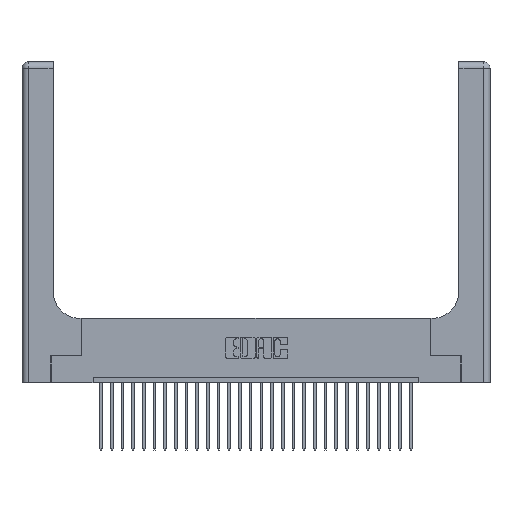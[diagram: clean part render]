
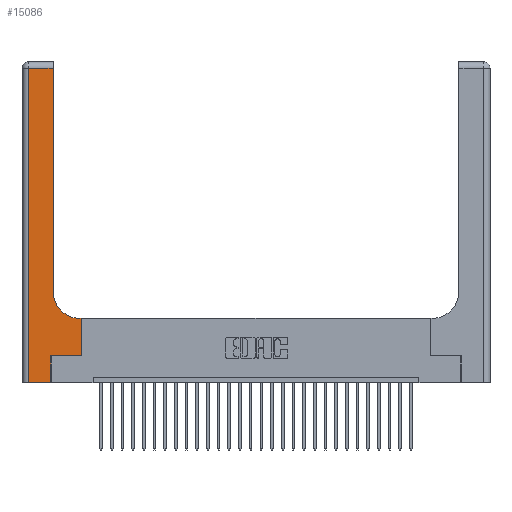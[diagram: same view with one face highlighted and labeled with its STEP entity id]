
A CAD part, top view. The second image highlights one B-rep face of the part: STEP entity #15086.
In plain terms, the highlighted planar face has unit normal (0, 0, 1).
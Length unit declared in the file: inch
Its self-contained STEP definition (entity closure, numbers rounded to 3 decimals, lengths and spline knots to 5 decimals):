
#100 = CARTESIAN_POINT ( 'NONE',  ( 0., 2.94, 0.37 ) ) ;
#261 = EDGE_CURVE ( 'NONE', #6286, #23740, #1936, .T. ) ;
#393 = DIRECTION ( 'NONE',  ( -1., 0., 0. ) ) ;
#439 = CARTESIAN_POINT ( 'NONE',  ( 0.5585, 0.6, 0.37 ) ) ;
#1012 = ORIENTED_EDGE ( 'NONE', *, *, #18084, .T. ) ;
#1936 = LINE ( 'NONE', #100, #5822 ) ;
#2536 = DIRECTION ( 'NONE',  ( 1., 0., 0. ) ) ;
#2660 = ORIENTED_EDGE ( 'NONE', *, *, #26138, .T. ) ;
#2692 = EDGE_CURVE ( 'NONE', #22903, #27558, #24898, .T. ) ;
#3680 = DIRECTION ( 'NONE',  ( -1., 0., 0. ) ) ;
#4266 = CARTESIAN_POINT ( 'NONE',  ( 0.269, 0., 0.37 ) ) ;
#4483 = EDGE_CURVE ( 'NONE', #23740, #28338, #14340, .T. ) ;
#4699 = DIRECTION ( 'NONE',  ( 0., 1., 0. ) ) ;
#4747 = EDGE_CURVE ( 'NONE', #27558, #6286, #4764, .T. ) ;
#4764 = LINE ( 'NONE', #18593, #23961 ) ;
#4982 = DIRECTION ( 'NONE',  ( -1., 0., 0. ) ) ;
#5817 = CARTESIAN_POINT ( 'NONE',  ( 0.2915, 0.85, 0.37 ) ) ;
#5822 = VECTOR ( 'NONE', #393, 39.37008 ) ;
#5964 = CARTESIAN_POINT ( 'NONE',  ( 0.06, 0., 0.37 ) ) ;
#6286 = VERTEX_POINT ( 'NONE', #26652 ) ;
#7009 = ORIENTED_EDGE ( 'NONE', *, *, #18083, .T. ) ;
#7066 = FACE_OUTER_BOUND ( 'NONE', #25324, .T. ) ;
#7945 = CARTESIAN_POINT ( 'NONE',  ( 0., 0., 0.37 ) ) ;
#8092 = CARTESIAN_POINT ( 'NONE',  ( 0.5585, 0.25, 0.37 ) ) ;
#8686 = CARTESIAN_POINT ( 'NONE',  ( 0.06, 2.94, 0.37 ) ) ;
#8848 = VERTEX_POINT ( 'NONE', #20283 ) ;
#9435 = CARTESIAN_POINT ( 'NONE',  ( 0.5585, 0.25, 0.37 ) ) ;
#9665 = DIRECTION ( 'NONE',  ( 0., 0., -1. ) ) ;
#9880 = ORIENTED_EDGE ( 'NONE', *, *, #25830, .T. ) ;
#11129 = ORIENTED_EDGE ( 'NONE', *, *, #2692, .T. ) ;
#11750 = DIRECTION ( 'NONE',  ( 0., 1., 0. ) ) ;
#11895 = PLANE ( 'NONE',  #16616 ) ;
#12113 = CARTESIAN_POINT ( 'NONE',  ( 0.269, 0.25, 0.37 ) ) ;
#13474 = VERTEX_POINT ( 'NONE', #23605 ) ;
#13719 = EDGE_CURVE ( 'NONE', #13474, #8848, #24953, .T. ) ;
#14340 = LINE ( 'NONE', #20123, #19332 ) ;
#15082 = VECTOR ( 'NONE', #28780, 39.37008 ) ;
#15086 = ADVANCED_FACE ( 'NONE', ( #7066 ), #11895, .F. ) ;
#15890 = VERTEX_POINT ( 'NONE', #9435 ) ;
#16402 = CARTESIAN_POINT ( 'NONE',  ( 0.5415, 0.85, 0.37 ) ) ;
#16513 = LINE ( 'NONE', #7945, #15082 ) ;
#16616 = AXIS2_PLACEMENT_3D ( 'NONE', #18836, #21236, #4982 ) ;
#16686 = ORIENTED_EDGE ( 'NONE', *, *, #4483, .T. ) ;
#17765 = VECTOR ( 'NONE', #24087, 39.37008 ) ;
#17891 = ORIENTED_EDGE ( 'NONE', *, *, #13719, .T. ) ;
#18083 = EDGE_CURVE ( 'NONE', #24902, #22903, #22198, .T. ) ;
#18084 = EDGE_CURVE ( 'NONE', #28338, #13474, #16513, .T. ) ;
#18593 = CARTESIAN_POINT ( 'NONE',  ( 0.2915, 3., 0.37 ) ) ;
#18836 = CARTESIAN_POINT ( 'NONE',  ( 0., 3., 0.37 ) ) ;
#19332 = VECTOR ( 'NONE', #24551, 39.37008 ) ;
#19511 = CARTESIAN_POINT ( 'NONE',  ( 0.5415, 0.6, 0.37 ) ) ;
#19600 = VECTOR ( 'NONE', #28011, 39.37008 ) ;
#20123 = CARTESIAN_POINT ( 'NONE',  ( 0.06, 3., 0.37 ) ) ;
#20283 = CARTESIAN_POINT ( 'NONE',  ( 0.269, 0.25, 0.37 ) ) ;
#20993 = VECTOR ( 'NONE', #4699, 39.37008 ) ;
#21236 = DIRECTION ( 'NONE',  ( 0., 0., -1. ) ) ;
#22198 = LINE ( 'NONE', #24352, #28598 ) ;
#22371 = LINE ( 'NONE', #8092, #17765 ) ;
#22868 = AXIS2_PLACEMENT_3D ( 'NONE', #16402, #9665, #2536 ) ;
#22903 = VERTEX_POINT ( 'NONE', #19511 ) ;
#23605 = CARTESIAN_POINT ( 'NONE',  ( 0.269, 0., 0.37 ) ) ;
#23740 = VERTEX_POINT ( 'NONE', #8686 ) ;
#23961 = VECTOR ( 'NONE', #11750, 39.37008 ) ;
#24087 = DIRECTION ( 'NONE',  ( 0., 1., 0. ) ) ;
#24352 = CARTESIAN_POINT ( 'NONE',  ( 0.2915, 0.6, 0.37 ) ) ;
#24551 = DIRECTION ( 'NONE',  ( 0., -1., 0. ) ) ;
#24675 = LINE ( 'NONE', #12113, #19600 ) ;
#24898 = CIRCLE ( 'NONE', #22868, 0.25 ) ;
#24902 = VERTEX_POINT ( 'NONE', #439 ) ;
#24953 = LINE ( 'NONE', #4266, #20993 ) ;
#25324 = EDGE_LOOP ( 'NONE', ( #29173, #25550, #16686, #1012, #17891, #2660, #9880, #7009, #11129 ) ) ;
#25550 = ORIENTED_EDGE ( 'NONE', *, *, #261, .T. ) ;
#25830 = EDGE_CURVE ( 'NONE', #15890, #24902, #22371, .T. ) ;
#26138 = EDGE_CURVE ( 'NONE', #8848, #15890, #24675, .T. ) ;
#26652 = CARTESIAN_POINT ( 'NONE',  ( 0.2915, 2.94, 0.37 ) ) ;
#27558 = VERTEX_POINT ( 'NONE', #5817 ) ;
#28011 = DIRECTION ( 'NONE',  ( 1., 0., 0. ) ) ;
#28338 = VERTEX_POINT ( 'NONE', #5964 ) ;
#28598 = VECTOR ( 'NONE', #3680, 39.37008 ) ;
#28780 = DIRECTION ( 'NONE',  ( 1., 0., 0. ) ) ;
#29173 = ORIENTED_EDGE ( 'NONE', *, *, #4747, .T. ) ;
